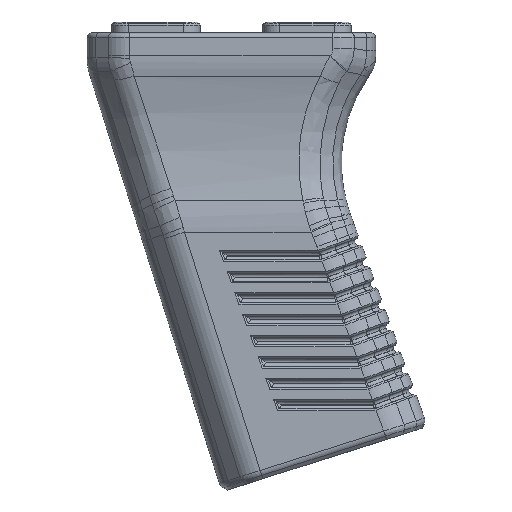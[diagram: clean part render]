
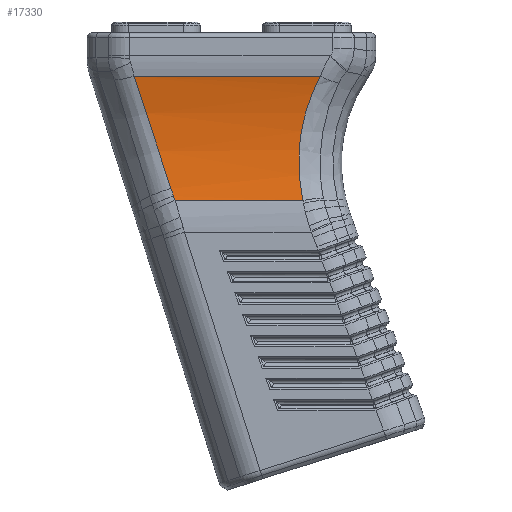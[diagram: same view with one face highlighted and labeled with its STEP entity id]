
A CAD part, left-side view. The second image highlights one B-rep face of the part: STEP entity #17330.
In plain terms, the highlighted cylindrical face has radius 37.604 mm (diameter 75.208 mm), a partial arc.
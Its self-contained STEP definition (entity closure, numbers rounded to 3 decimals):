
#328=CYLINDRICAL_SURFACE('',#19063,37.604);
#1580=LINE('',#33023,#2797);
#1581=LINE('',#33025,#2798);
#2797=VECTOR('',#23429,10.);
#2798=VECTOR('',#23432,10.);
#4335=FACE_OUTER_BOUND('',#5453,.T.);
#5453=EDGE_LOOP('',(#15189,#15190,#15191,#15192,#15193,#15194));
#5937=B_SPLINE_CURVE_WITH_KNOTS('',3,(#31761,#31762,#31763,#31764),
 .UNSPECIFIED.,.F.,.F.,(4,4),(0.,1.726),
 .UNSPECIFIED.);
#5938=B_SPLINE_CURVE_WITH_KNOTS('',3,(#31782,#31783,#31784,#31785),
 .UNSPECIFIED.,.F.,.F.,(4,4),(0.,0.118),
 .UNSPECIFIED.);
#5946=B_SPLINE_CURVE_WITH_KNOTS('',3,(#31906,#31907,#31908,#31909),
 .UNSPECIFIED.,.F.,.F.,(4,4),(0.,0.067),.UNSPECIFIED.);
#5999=B_SPLINE_CURVE_WITH_KNOTS('',3,(#32937,#32938,#32939,#32940,#32941),
 .UNSPECIFIED.,.F.,.F.,(4,1,4),(0.,0.805,1.879),
 .UNSPECIFIED.);
#8136=VERTEX_POINT('',#31694);
#8139=VERTEX_POINT('',#31723);
#8140=VERTEX_POINT('',#31781);
#8145=VERTEX_POINT('',#31852);
#8194=VERTEX_POINT('',#32934);
#8195=VERTEX_POINT('',#32936);
#10481=EDGE_CURVE('',#8136,#8139,#5937,.T.);
#10482=EDGE_CURVE('',#8139,#8140,#5938,.T.);
#10493=EDGE_CURVE('',#8140,#8145,#5946,.T.);
#10583=EDGE_CURVE('',#8195,#8194,#5999,.T.);
#10590=EDGE_CURVE('',#8194,#8136,#1580,.T.);
#10591=EDGE_CURVE('',#8145,#8195,#1581,.T.);
#15189=ORIENTED_EDGE('',*,*,#10481,.T.);
#15190=ORIENTED_EDGE('',*,*,#10482,.T.);
#15191=ORIENTED_EDGE('',*,*,#10493,.T.);
#15192=ORIENTED_EDGE('',*,*,#10591,.T.);
#15193=ORIENTED_EDGE('',*,*,#10583,.T.);
#15194=ORIENTED_EDGE('',*,*,#10590,.T.);
#17330=ADVANCED_FACE('',(#4335),#328,.F.);
#19063=AXIS2_PLACEMENT_3D('',#33024,#23430,#23431);
#23429=DIRECTION('',(0.,1.,0.));
#23430=DIRECTION('center_axis',(0.,-1.,0.));
#23431=DIRECTION('ref_axis',(0.966,0.,0.26));
#23432=DIRECTION('',(0.,-1.,0.));
#31694=CARTESIAN_POINT('',(-10.588,-132.352,97.275));
#31723=CARTESIAN_POINT('',(-10.15,-137.223,82.415));
#31761=CARTESIAN_POINT('Ctrl Pts',(-10.588,-132.352,
97.275));
#31762=CARTESIAN_POINT('Ctrl Pts',(-9.457,-133.959,92.412));
#31763=CARTESIAN_POINT('Ctrl Pts',(-9.308,-135.622,87.338));
#31764=CARTESIAN_POINT('Ctrl Pts',(-10.15,-137.223,
82.415));
#31781=CARTESIAN_POINT('',(-10.336,-137.565,81.411));
#31782=CARTESIAN_POINT('Ctrl Pts',(-10.15,-137.223,
82.415));
#31783=CARTESIAN_POINT('Ctrl Pts',(-10.208,-137.333,
82.078));
#31784=CARTESIAN_POINT('Ctrl Pts',(-10.27,-137.447,
81.744));
#31785=CARTESIAN_POINT('Ctrl Pts',(-10.336,-137.565,81.411));
#31852=CARTESIAN_POINT('',(-10.452,-137.783,80.85));
#31906=CARTESIAN_POINT('Ctrl Pts',(-10.336,-137.565,
81.411));
#31907=CARTESIAN_POINT('Ctrl Pts',(-10.374,-137.633,
81.222));
#31908=CARTESIAN_POINT('Ctrl Pts',(-10.413,-137.705,81.035));
#31909=CARTESIAN_POINT('Ctrl Pts',(-10.452,-137.783,
80.85));
#32934=CARTESIAN_POINT('',(-10.588,-157.023,97.275));
#32936=CARTESIAN_POINT('',(-10.452,-154.693,80.85));
#32937=CARTESIAN_POINT('Ctrl Pts',(-10.452,-154.693,80.85));
#32938=CARTESIAN_POINT('Ctrl Pts',(-9.952,-154.18,
83.178));
#32939=CARTESIAN_POINT('Ctrl Pts',(-9.28,-153.808,
88.874));
#32940=CARTESIAN_POINT('Ctrl Pts',(-9.928,-155.475,
94.435));
#32941=CARTESIAN_POINT('Ctrl Pts',(-10.588,-157.023,
97.275));
#33023=CARTESIAN_POINT('',(-10.588,-164.329,97.275));
#33024=CARTESIAN_POINT('Origin',(-47.215,-164.329,88.76));
#33025=CARTESIAN_POINT('',(-10.452,-164.329,80.85));
